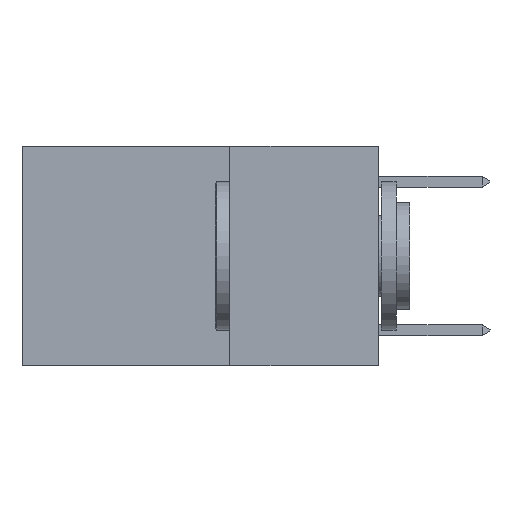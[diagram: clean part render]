
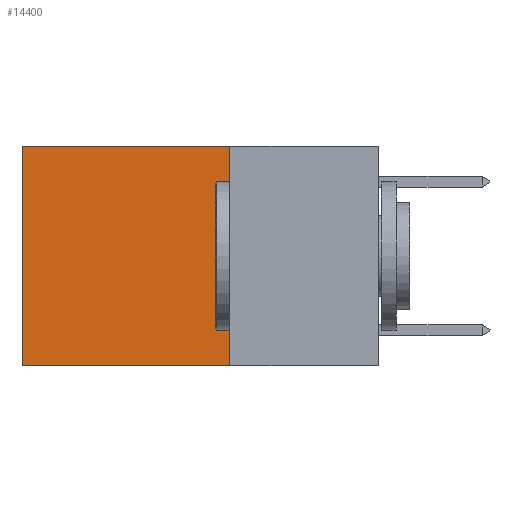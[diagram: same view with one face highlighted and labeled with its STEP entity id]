
A CAD part, left-side view. The second image highlights one B-rep face of the part: STEP entity #14400.
In plain terms, the highlighted planar face has unit normal (-1, 0, 0).
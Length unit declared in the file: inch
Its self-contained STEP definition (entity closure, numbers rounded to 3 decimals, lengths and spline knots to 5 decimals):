
#698 = EDGE_CURVE ( 'NONE', #2209, #5034, #16276, .T. ) ;
#1242 = VECTOR ( 'NONE', #4572, 39.37008 ) ;
#2209 = VERTEX_POINT ( 'NONE', #20408 ) ;
#2924 = CARTESIAN_POINT ( 'NONE',  ( 0.2625, 0.25, 0. ) ) ;
#3144 = ORIENTED_EDGE ( 'NONE', *, *, #9410, .T. ) ;
#4370 = EDGE_LOOP ( 'NONE', ( #7085, #7632, #13321, #3144 ) ) ;
#4572 = DIRECTION ( 'NONE',  ( 0., 0., -1. ) ) ;
#5034 = VERTEX_POINT ( 'NONE', #15166 ) ;
#6348 = CARTESIAN_POINT ( 'NONE',  ( 0.2625, 0.25, 0. ) ) ;
#7085 = ORIENTED_EDGE ( 'NONE', *, *, #9172, .T. ) ;
#7445 = DIRECTION ( 'NONE',  ( 1., 0., 0. ) ) ;
#7632 = ORIENTED_EDGE ( 'NONE', *, *, #8028, .F. ) ;
#7671 = DIRECTION ( 'NONE',  ( 0., 0., -1. ) ) ;
#8028 = EDGE_CURVE ( 'NONE', #5034, #12892, #12638, .T. ) ;
#8086 = CARTESIAN_POINT ( 'NONE',  ( 0.2625, 0.25, -0.37 ) ) ;
#8599 = CARTESIAN_POINT ( 'NONE',  ( 0.2625, 0.6, -0.37 ) ) ;
#9172 = EDGE_CURVE ( 'NONE', #11574, #12892, #18016, .T. ) ;
#9410 = EDGE_CURVE ( 'NONE', #2209, #11574, #14928, .T. ) ;
#10872 = CARTESIAN_POINT ( 'NONE',  ( 0.2625, 0.25, 0. ) ) ;
#11574 = VERTEX_POINT ( 'NONE', #14964 ) ;
#11894 = VECTOR ( 'NONE', #16428, 39.37008 ) ;
#12638 = LINE ( 'NONE', #8086, #11894 ) ;
#12892 = VERTEX_POINT ( 'NONE', #8599 ) ;
#13321 = ORIENTED_EDGE ( 'NONE', *, *, #698, .F. ) ;
#14400 = ADVANCED_FACE ( 'NONE', ( #20310 ), #17547, .F. ) ;
#14928 = LINE ( 'NONE', #6348, #20377 ) ;
#14964 = CARTESIAN_POINT ( 'NONE',  ( 0.2625, 0.6, 0. ) ) ;
#15166 = CARTESIAN_POINT ( 'NONE',  ( 0.2625, 0.25, -0.37 ) ) ;
#16276 = LINE ( 'NONE', #2924, #1242 ) ;
#16428 = DIRECTION ( 'NONE',  ( 0., 1., 0. ) ) ;
#17547 = PLANE ( 'NONE',  #21416 ) ;
#17793 = VECTOR ( 'NONE', #7671, 39.37008 ) ;
#18016 = LINE ( 'NONE', #19133, #17793 ) ;
#18976 = DIRECTION ( 'NONE',  ( 0., 0., -1. ) ) ;
#19133 = CARTESIAN_POINT ( 'NONE',  ( 0.2625, 0.6, 0. ) ) ;
#19345 = DIRECTION ( 'NONE',  ( 0., 1., 0. ) ) ;
#20310 = FACE_OUTER_BOUND ( 'NONE', #4370, .T. ) ;
#20377 = VECTOR ( 'NONE', #19345, 39.37008 ) ;
#20408 = CARTESIAN_POINT ( 'NONE',  ( 0.2625, 0.25, 0. ) ) ;
#21416 = AXIS2_PLACEMENT_3D ( 'NONE', #10872, #7445, #18976 ) ;
